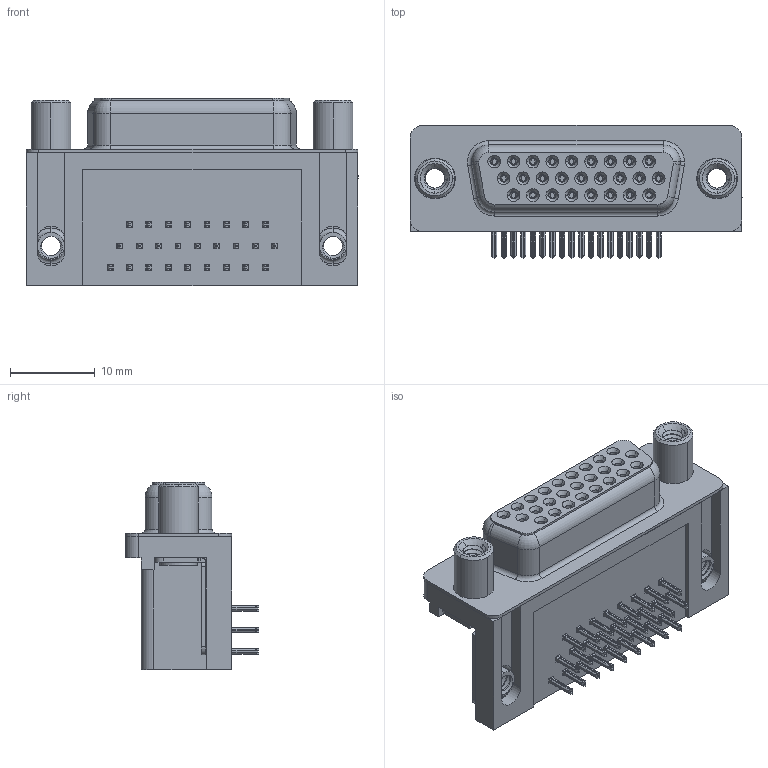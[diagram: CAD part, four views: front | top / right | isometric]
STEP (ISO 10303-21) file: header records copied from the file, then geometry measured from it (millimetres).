
FILE_DESCRIPTION (( 'STEP AP203' ), '1' );
FILE_NAME ('634-026-663-050.STEP', '2018-11-09T23:59:22', ( '' ), ( '' ), 'SwSTEP 2.0', 'SolidWorks 2016', '' );
FILE_SCHEMA (( 'CONFIG_CONTROL_DESIGN' ));
Length unit declared in the file: millimetre
Products named in the file (8): 634-026-663-050; 634 Housing_26 Socket; 634 Shell_26 Socket; Contact Bottom; Contact Middle; Contact Top; 4-40 Threaded Board Mount; Round Threaded Standoff
Assembly tree (32 placements, depth 2):
  634-026-663-050
    634 Housing_26 Socket
    634 Shell_26 Socket
    Contact Bottom  x8
    Contact Middle  x9
    Contact Top  x9
    4-40 Threaded Board Mount  x2
    Round Threaded Standoff  x2
Bounding box: 39.22 x 15.73 x 22.1 mm (x, y, z)
Volume: 6468.1 mm3; surface area: 9358.8 mm2
Topology: 32 solids, 32 shells, 4005 faces, 10546 edges, 6630 vertices
Faces by surface type: plane 1763, cylinder 958, bspline 926, cone 324, torus 34
Entity records: 38700 total; most frequent: CARTESIAN_POINT 13978, ORIENTED_EDGE 5040, DIRECTION 4388, EDGE_CURVE 2520, VERTEX_POINT 1608, LINE 1574, VECTOR 1574, AXIS2_PLACEMENT_3D 1407
